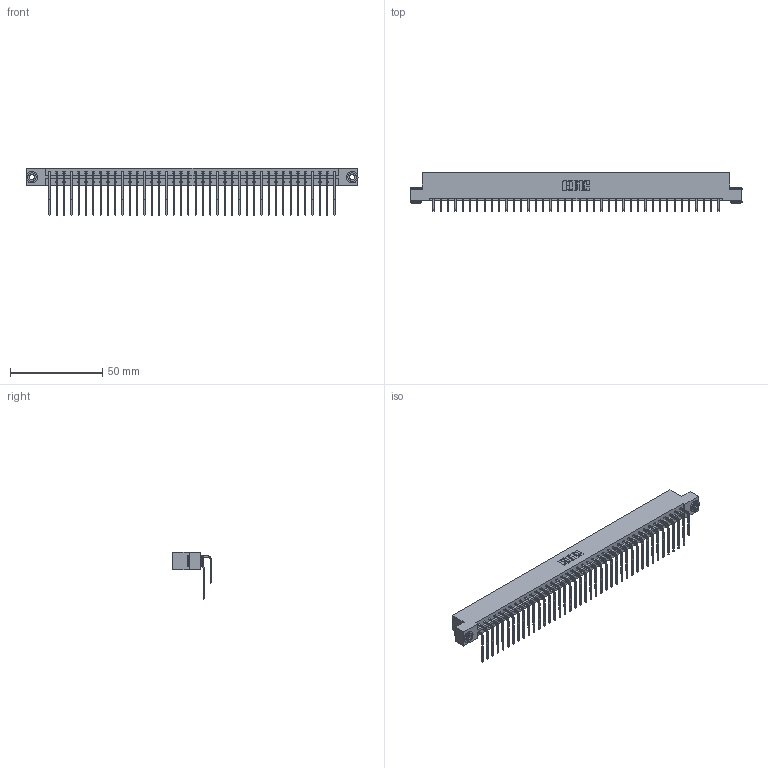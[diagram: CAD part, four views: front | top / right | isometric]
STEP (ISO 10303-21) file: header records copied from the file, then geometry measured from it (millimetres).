
FILE_DESCRIPTION (( 'STEP AP203' ), '1' );
FILE_NAME ('833-080-559-203.STEP', '2020-06-05T22:37:09', ( '' ), ( '' ), 'SwSTEP 2.0', 'SolidWorks 2020', '' );
FILE_SCHEMA (( 'CONFIG_CONTROL_DESIGN' ));
Length unit declared in the file: inch
Products named in the file (5): 345-292-001_559 Tail - 2; 833-080-559-203; 345-250-002_345-250-002-102; 833 Part_Flush - .156 Dia - TH; 345-292-001_558 559 Tail - 1
Assembly tree (83 placements, depth 2):
  833-080-559-203
    833 Part_Flush - .156 Dia - TH
    345-292-001_558 559 Tail - 1  x40
    345-292-001_559 Tail - 2  x40
    345-250-002_345-250-002-102  x2
Bounding box: 180.04 x 20.9 x 25.53 mm (x, y, z)
Volume: 18842.8 mm3; surface area: 24775 mm2
Topology: 83 solids, 83 shells, 4472 faces, 13267 edges, 8734 vertices
Faces by surface type: plane 3120, cylinder 1344, cone 8
Entity records: 28426 total; most frequent: CARTESIAN_POINT 4740, ORIENTED_EDGE 4618, DIRECTION 4067, EDGE_CURVE 2309, LINE 2117, VECTOR 2117, VERTEX_POINT 1534, AXIS2_PLACEMENT_3D 975
